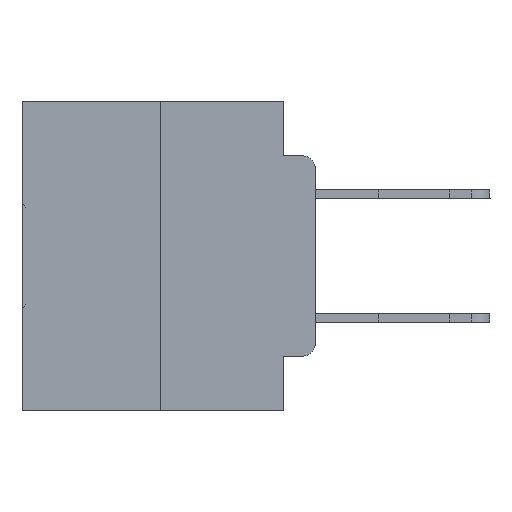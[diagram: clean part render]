
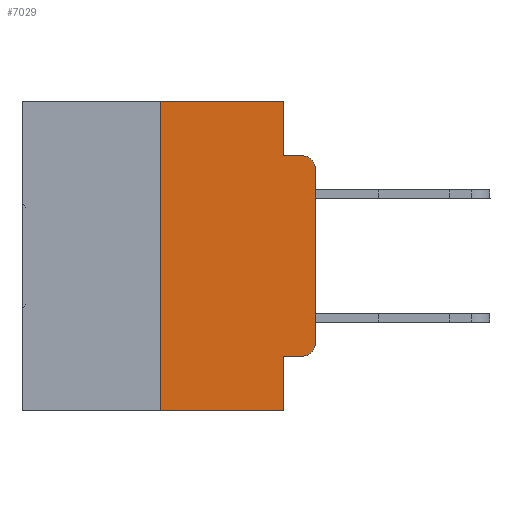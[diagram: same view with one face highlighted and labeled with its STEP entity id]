
A CAD part, left-side view. The second image highlights one B-rep face of the part: STEP entity #7029.
In plain terms, the highlighted planar face has unit normal (-1, 0, 0).
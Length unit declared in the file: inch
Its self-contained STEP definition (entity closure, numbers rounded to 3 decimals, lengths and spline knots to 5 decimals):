
#27 = VECTOR ( 'NONE', #3696, 39.37008 ) ;
#445 = EDGE_CURVE ( 'NONE', #1356, #12647, #23554, .T. ) ;
#622 = CARTESIAN_POINT ( 'NONE',  ( 0., 0.051, -0.4115 ) ) ;
#704 = ORIENTED_EDGE ( 'NONE', *, *, #30643, .F. ) ;
#901 = EDGE_CURVE ( 'NONE', #3906, #16360, #15805, .T. ) ;
#1356 = VERTEX_POINT ( 'NONE', #5240 ) ;
#2367 = DIRECTION ( 'NONE',  ( 0., 0., -1. ) ) ;
#2587 = CARTESIAN_POINT ( 'NONE',  ( 0., 0.02, -0.3915 ) ) ;
#3062 = LINE ( 'NONE', #19127, #28213 ) ;
#3621 = CARTESIAN_POINT ( 'NONE',  ( 0., 0.051, -0.0885 ) ) ;
#3696 = DIRECTION ( 'NONE',  ( 0., -1., 0. ) ) ;
#3906 = VERTEX_POINT ( 'NONE', #14530 ) ;
#4277 = VECTOR ( 'NONE', #25256, 39.37008 ) ;
#4478 = CARTESIAN_POINT ( 'NONE',  ( 0., 0.051, 0. ) ) ;
#4967 = CARTESIAN_POINT ( 'NONE',  ( 0., 0.473, -0.5 ) ) ;
#5224 = DIRECTION ( 'NONE',  ( 0., 0., -1. ) ) ;
#5240 = CARTESIAN_POINT ( 'NONE',  ( 0., 0., -0.1085 ) ) ;
#5742 = EDGE_CURVE ( 'NONE', #21727, #1356, #27503, .T. ) ;
#6295 = CARTESIAN_POINT ( 'NONE',  ( 0., 0., -0.3915 ) ) ;
#6330 = CARTESIAN_POINT ( 'NONE',  ( 0., 0.473, 0. ) ) ;
#6793 = CIRCLE ( 'NONE', #7041, 0.02 ) ;
#7029 = ADVANCED_FACE ( 'NONE', ( #7559 ), #23091, .F. ) ;
#7041 = AXIS2_PLACEMENT_3D ( 'NONE', #2587, #20816, #5224 ) ;
#7267 = ORIENTED_EDGE ( 'NONE', *, *, #5742, .T. ) ;
#7559 = FACE_OUTER_BOUND ( 'NONE', #9362, .T. ) ;
#8017 = CARTESIAN_POINT ( 'NONE',  ( 0., 0.051, 0. ) ) ;
#8523 = ORIENTED_EDGE ( 'NONE', *, *, #16847, .T. ) ;
#8864 = CARTESIAN_POINT ( 'NONE',  ( 0., 0.02, -0.0885 ) ) ;
#9048 = LINE ( 'NONE', #18440, #22092 ) ;
#9308 = ORIENTED_EDGE ( 'NONE', *, *, #28938, .F. ) ;
#9362 = EDGE_LOOP ( 'NONE', ( #7267, #19080, #32668, #704, #29133, #9308, #24743, #31522, #27580, #8523 ) ) ;
#9459 = VERTEX_POINT ( 'NONE', #16484 ) ;
#10661 = VERTEX_POINT ( 'NONE', #8017 ) ;
#11343 = LINE ( 'NONE', #18768, #24337 ) ;
#12027 = LINE ( 'NONE', #4478, #4277 ) ;
#12647 = VERTEX_POINT ( 'NONE', #8864 ) ;
#12978 = LINE ( 'NONE', #18147, #25942 ) ;
#13937 = VERTEX_POINT ( 'NONE', #14635 ) ;
#13946 = LINE ( 'NONE', #6330, #27 ) ;
#14530 = CARTESIAN_POINT ( 'NONE',  ( 0., 0.25, -0.5 ) ) ;
#14635 = CARTESIAN_POINT ( 'NONE',  ( 0., 0.02, -0.4115 ) ) ;
#15805 = LINE ( 'NONE', #4967, #28717 ) ;
#16360 = VERTEX_POINT ( 'NONE', #18904 ) ;
#16484 = CARTESIAN_POINT ( 'NONE',  ( 0., 0.25, 0. ) ) ;
#16847 = EDGE_CURVE ( 'NONE', #13937, #21727, #6793, .T. ) ;
#17157 = DIRECTION ( 'NONE',  ( -1., 0., 0. ) ) ;
#17426 = DIRECTION ( 'NONE',  ( 0., 0., -1. ) ) ;
#17457 = CARTESIAN_POINT ( 'NONE',  ( 0., 0.02, -0.1085 ) ) ;
#17992 = DIRECTION ( 'NONE',  ( 1., 0., 0. ) ) ;
#18147 = CARTESIAN_POINT ( 'NONE',  ( 0., 0.051, -0.4115 ) ) ;
#18440 = CARTESIAN_POINT ( 'NONE',  ( 0., 0.051, -0.0885 ) ) ;
#18768 = CARTESIAN_POINT ( 'NONE',  ( 0., 0.25, 0. ) ) ;
#18904 = CARTESIAN_POINT ( 'NONE',  ( 0., 0.051, -0.5 ) ) ;
#19033 = VECTOR ( 'NONE', #19971, 39.37008 ) ;
#19080 = ORIENTED_EDGE ( 'NONE', *, *, #445, .T. ) ;
#19127 = CARTESIAN_POINT ( 'NONE',  ( 0., 0.051, 0. ) ) ;
#19688 = DIRECTION ( 'NONE',  ( 0., -1., 0. ) ) ;
#19971 = DIRECTION ( 'NONE',  ( 0., 0., 1. ) ) ;
#20529 = VERTEX_POINT ( 'NONE', #3621 ) ;
#20748 = DIRECTION ( 'NONE',  ( 0., -1., 0. ) ) ;
#20816 = DIRECTION ( 'NONE',  ( -1., 0., 0. ) ) ;
#21047 = DIRECTION ( 'NONE',  ( 0., -1., 0. ) ) ;
#21384 = DIRECTION ( 'NONE',  ( 0., 0., 1. ) ) ;
#21727 = VERTEX_POINT ( 'NONE', #6295 ) ;
#22074 = EDGE_CURVE ( 'NONE', #25635, #13937, #12978, .T. ) ;
#22092 = VECTOR ( 'NONE', #21047, 39.37008 ) ;
#23027 = AXIS2_PLACEMENT_3D ( 'NONE', #17457, #17157, #17426 ) ;
#23091 = PLANE ( 'NONE',  #31100 ) ;
#23554 = CIRCLE ( 'NONE', #23027, 0.02 ) ;
#23803 = EDGE_CURVE ( 'NONE', #25635, #16360, #3062, .T. ) ;
#24337 = VECTOR ( 'NONE', #21384, 39.37008 ) ;
#24743 = ORIENTED_EDGE ( 'NONE', *, *, #901, .T. ) ;
#25256 = DIRECTION ( 'NONE',  ( 0., 0., -1. ) ) ;
#25635 = VERTEX_POINT ( 'NONE', #622 ) ;
#25942 = VECTOR ( 'NONE', #20748, 39.37008 ) ;
#26785 = DIRECTION ( 'NONE',  ( 0., 0., -1. ) ) ;
#27503 = LINE ( 'NONE', #30283, #19033 ) ;
#27580 = ORIENTED_EDGE ( 'NONE', *, *, #22074, .T. ) ;
#28213 = VECTOR ( 'NONE', #26785, 39.37008 ) ;
#28717 = VECTOR ( 'NONE', #19688, 39.37008 ) ;
#28938 = EDGE_CURVE ( 'NONE', #3906, #9459, #11343, .T. ) ;
#29133 = ORIENTED_EDGE ( 'NONE', *, *, #32551, .F. ) ;
#30283 = CARTESIAN_POINT ( 'NONE',  ( 0., 0., 0. ) ) ;
#30643 = EDGE_CURVE ( 'NONE', #10661, #20529, #12027, .T. ) ;
#31100 = AXIS2_PLACEMENT_3D ( 'NONE', #33284, #17992, #2367 ) ;
#31522 = ORIENTED_EDGE ( 'NONE', *, *, #23803, .F. ) ;
#32312 = EDGE_CURVE ( 'NONE', #20529, #12647, #9048, .T. ) ;
#32551 = EDGE_CURVE ( 'NONE', #9459, #10661, #13946, .T. ) ;
#32668 = ORIENTED_EDGE ( 'NONE', *, *, #32312, .F. ) ;
#33284 = CARTESIAN_POINT ( 'NONE',  ( 0., 0.473, 0. ) ) ;
